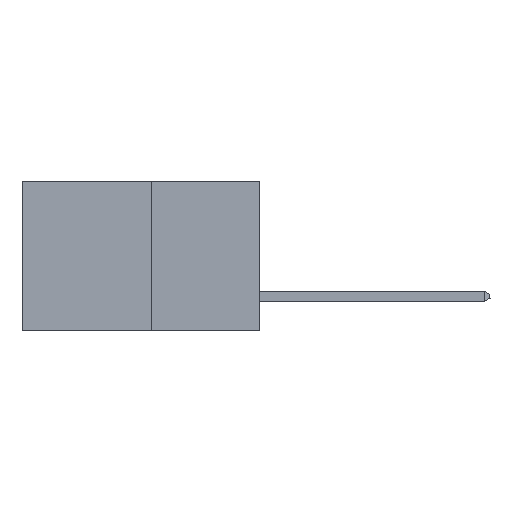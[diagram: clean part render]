
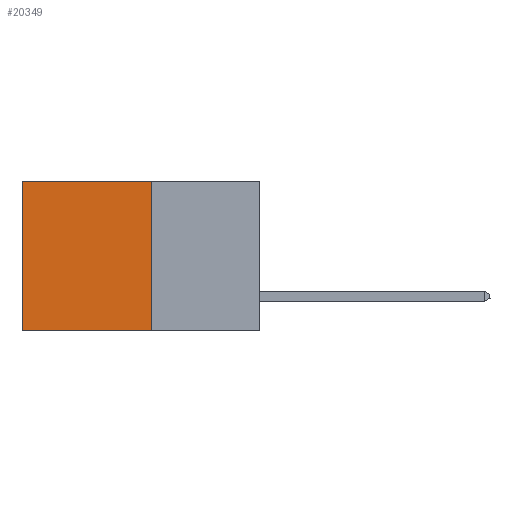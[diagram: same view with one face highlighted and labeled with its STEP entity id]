
A CAD part, left-side view. The second image highlights one B-rep face of the part: STEP entity #20349.
In plain terms, the highlighted planar face has unit normal (-1, 0, 0).
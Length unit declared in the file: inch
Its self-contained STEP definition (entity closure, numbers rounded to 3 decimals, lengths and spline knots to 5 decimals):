
#351 = CARTESIAN_POINT ( 'NONE',  ( 0.277, 0.27, -0.37 ) ) ;
#632 = ORIENTED_EDGE ( 'NONE', *, *, #30791, .T. ) ;
#1954 = FACE_OUTER_BOUND ( 'NONE', #20286, .T. ) ;
#2017 = DIRECTION ( 'NONE',  ( 0., 0., -1. ) ) ;
#2964 = AXIS2_PLACEMENT_3D ( 'NONE', #24706, #29673, #14774 ) ;
#3172 = ORIENTED_EDGE ( 'NONE', *, *, #29999, .T. ) ;
#4489 = EDGE_CURVE ( 'NONE', #31401, #8572, #21083, .T. ) ;
#5221 = ORIENTED_EDGE ( 'NONE', *, *, #32153, .F. ) ;
#7789 = VECTOR ( 'NONE', #2017, 39.37008 ) ;
#7832 = CARTESIAN_POINT ( 'NONE',  ( 0.277, 0.27, 0. ) ) ;
#8413 = CARTESIAN_POINT ( 'NONE',  ( 0.277, 0.27, -0.37 ) ) ;
#8572 = VERTEX_POINT ( 'NONE', #8413 ) ;
#9905 = CARTESIAN_POINT ( 'NONE',  ( 0.277, 0.59, -0.37 ) ) ;
#12131 = VECTOR ( 'NONE', #27333, 39.37008 ) ;
#12523 = VERTEX_POINT ( 'NONE', #24648 ) ;
#12708 = CARTESIAN_POINT ( 'NONE',  ( 0.277, 0.59, 0. ) ) ;
#12843 = VECTOR ( 'NONE', #25346, 39.37008 ) ;
#13627 = LINE ( 'NONE', #22829, #12843 ) ;
#14774 = DIRECTION ( 'NONE',  ( 0., 0., -1. ) ) ;
#15322 = VECTOR ( 'NONE', #30441, 39.37008 ) ;
#15577 = VERTEX_POINT ( 'NONE', #12708 ) ;
#20286 = EDGE_LOOP ( 'NONE', ( #3172, #5221, #29062, #632 ) ) ;
#20349 = ADVANCED_FACE ( 'NONE', ( #1954 ), #27203, .F. ) ;
#21083 = LINE ( 'NONE', #351, #7789 ) ;
#22829 = CARTESIAN_POINT ( 'NONE',  ( 0.277, 0.27, 0. ) ) ;
#22970 = CARTESIAN_POINT ( 'NONE',  ( 0.277, 0.27, -0.37 ) ) ;
#23504 = LINE ( 'NONE', #22970, #15322 ) ;
#24648 = CARTESIAN_POINT ( 'NONE',  ( 0.277, 0.59, -0.37 ) ) ;
#24706 = CARTESIAN_POINT ( 'NONE',  ( 0.277, 0.27, -0.37 ) ) ;
#25346 = DIRECTION ( 'NONE',  ( 0., 1., 0. ) ) ;
#25378 = LINE ( 'NONE', #9905, #12131 ) ;
#27203 = PLANE ( 'NONE',  #2964 ) ;
#27333 = DIRECTION ( 'NONE',  ( 0., 0., -1. ) ) ;
#29062 = ORIENTED_EDGE ( 'NONE', *, *, #4489, .F. ) ;
#29673 = DIRECTION ( 'NONE',  ( 1., 0., 0. ) ) ;
#29999 = EDGE_CURVE ( 'NONE', #15577, #12523, #25378, .T. ) ;
#30441 = DIRECTION ( 'NONE',  ( 0., 1., 0. ) ) ;
#30791 = EDGE_CURVE ( 'NONE', #31401, #15577, #13627, .T. ) ;
#31401 = VERTEX_POINT ( 'NONE', #7832 ) ;
#32153 = EDGE_CURVE ( 'NONE', #8572, #12523, #23504, .T. ) ;
